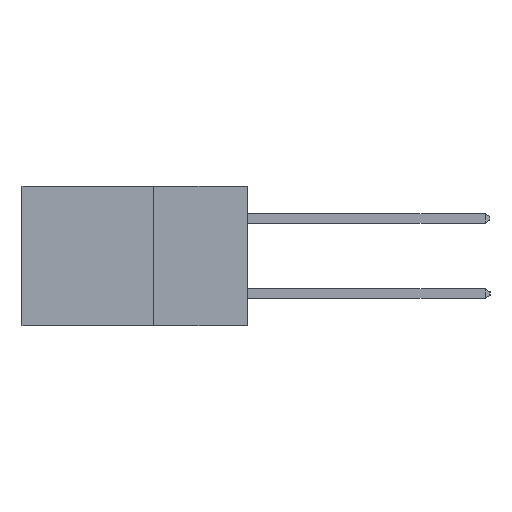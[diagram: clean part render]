
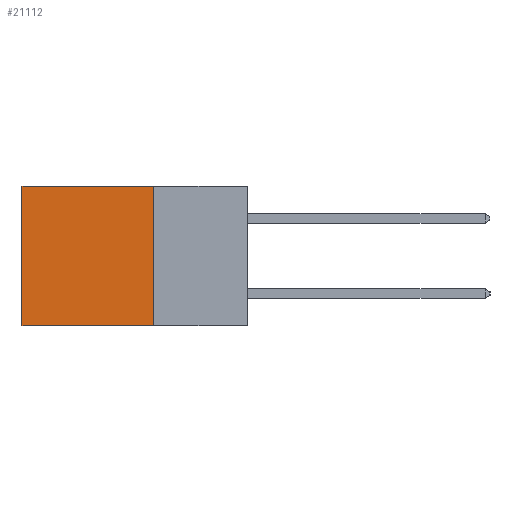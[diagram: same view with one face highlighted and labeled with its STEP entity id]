
A CAD part, left-side view. The second image highlights one B-rep face of the part: STEP entity #21112.
In plain terms, the highlighted planar face has unit normal (-1, 0, 0).
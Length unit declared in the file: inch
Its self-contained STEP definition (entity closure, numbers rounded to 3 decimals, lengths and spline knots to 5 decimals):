
#185 = ORIENTED_EDGE ( 'NONE', *, *, #25491, .T. ) ;
#241 = LINE ( 'NONE', #19610, #25232 ) ;
#440 = DIRECTION ( 'NONE',  ( 0., 0., -1. ) ) ;
#838 = CARTESIAN_POINT ( 'NONE',  ( 0.2615, 0.6, 0. ) ) ;
#2084 = CARTESIAN_POINT ( 'NONE',  ( 0.2615, 0.6, -0.37 ) ) ;
#2583 = CARTESIAN_POINT ( 'NONE',  ( 0.2615, 0.6, -0.37 ) ) ;
#3387 = AXIS2_PLACEMENT_3D ( 'NONE', #10502, #12503, #440 ) ;
#4844 = CARTESIAN_POINT ( 'NONE',  ( 0.2615, 0.25, -0.37 ) ) ;
#6884 = DIRECTION ( 'NONE',  ( 0., 1., 0. ) ) ;
#7224 = LINE ( 'NONE', #7759, #17157 ) ;
#7759 = CARTESIAN_POINT ( 'NONE',  ( 0.2615, 0.25, 0. ) ) ;
#8252 = ORIENTED_EDGE ( 'NONE', *, *, #16891, .F. ) ;
#8483 = PLANE ( 'NONE',  #3387 ) ;
#8630 = VERTEX_POINT ( 'NONE', #19952 ) ;
#8748 = VECTOR ( 'NONE', #6884, 39.37008 ) ;
#8898 = VERTEX_POINT ( 'NONE', #838 ) ;
#9198 = LINE ( 'NONE', #2084, #18445 ) ;
#9790 = DIRECTION ( 'NONE',  ( 0., 1., 0. ) ) ;
#10150 = EDGE_CURVE ( 'NONE', #24527, #23154, #19213, .T. ) ;
#10502 = CARTESIAN_POINT ( 'NONE',  ( 0.2615, 0.25, -0.37 ) ) ;
#12503 = DIRECTION ( 'NONE',  ( 1., 0., 0. ) ) ;
#13828 = DIRECTION ( 'NONE',  ( 0., 0., -1. ) ) ;
#14527 = ORIENTED_EDGE ( 'NONE', *, *, #15156, .T. ) ;
#15156 = EDGE_CURVE ( 'NONE', #8898, #23154, #9198, .T. ) ;
#16072 = FACE_OUTER_BOUND ( 'NONE', #17605, .T. ) ;
#16891 = EDGE_CURVE ( 'NONE', #8630, #24527, #241, .T. ) ;
#17157 = VECTOR ( 'NONE', #9790, 39.37008 ) ;
#17605 = EDGE_LOOP ( 'NONE', ( #14527, #23466, #8252, #185 ) ) ;
#18445 = VECTOR ( 'NONE', #21864, 39.37008 ) ;
#19213 = LINE ( 'NONE', #4844, #8748 ) ;
#19610 = CARTESIAN_POINT ( 'NONE',  ( 0.2615, 0.25, -0.37 ) ) ;
#19952 = CARTESIAN_POINT ( 'NONE',  ( 0.2615, 0.25, 0. ) ) ;
#21112 = ADVANCED_FACE ( 'NONE', ( #16072 ), #8483, .F. ) ;
#21864 = DIRECTION ( 'NONE',  ( 0., 0., -1. ) ) ;
#22205 = CARTESIAN_POINT ( 'NONE',  ( 0.2615, 0.25, -0.37 ) ) ;
#23154 = VERTEX_POINT ( 'NONE', #2583 ) ;
#23466 = ORIENTED_EDGE ( 'NONE', *, *, #10150, .F. ) ;
#24527 = VERTEX_POINT ( 'NONE', #22205 ) ;
#25232 = VECTOR ( 'NONE', #13828, 39.37008 ) ;
#25491 = EDGE_CURVE ( 'NONE', #8630, #8898, #7224, .T. ) ;
